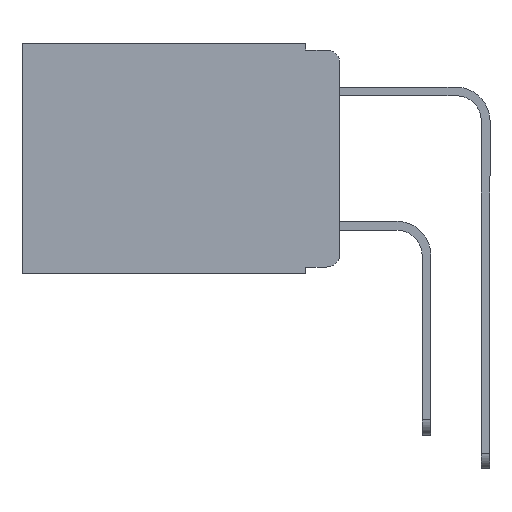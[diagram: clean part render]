
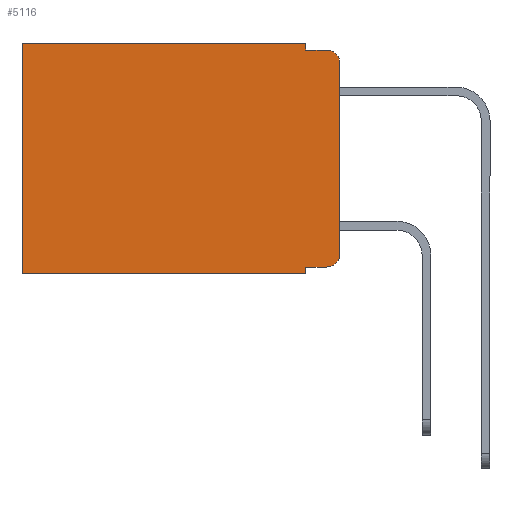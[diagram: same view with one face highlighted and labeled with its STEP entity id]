
A CAD part, left-side view. The second image highlights one B-rep face of the part: STEP entity #5116.
In plain terms, the highlighted planar face has unit normal (-1, 0, 0).
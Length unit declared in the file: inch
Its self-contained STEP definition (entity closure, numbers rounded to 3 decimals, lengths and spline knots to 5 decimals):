
#113 = EDGE_LOOP ( 'NONE', ( #5442, #7482, #9654, #10211, #340, #6336, #5883, #1117, #10622, #8975 ) ) ;
#290 = CARTESIAN_POINT ( 'NONE',  ( 0.298, 0.02, -0.333 ) ) ;
#305 = DIRECTION ( 'NONE',  ( 0., 0., -1. ) ) ;
#340 = ORIENTED_EDGE ( 'NONE', *, *, #9689, .T. ) ;
#457 = VERTEX_POINT ( 'NONE', #6332 ) ;
#502 = VERTEX_POINT ( 'NONE', #6420 ) ;
#534 = DIRECTION ( 'NONE',  ( 0., 1., 0. ) ) ;
#562 = CARTESIAN_POINT ( 'NONE',  ( 0.298, 0., -0.03 ) ) ;
#563 = CARTESIAN_POINT ( 'NONE',  ( 0.298, 0.051, -0.333 ) ) ;
#743 = VERTEX_POINT ( 'NONE', #6463 ) ;
#768 = LINE ( 'NONE', #3056, #7172 ) ;
#877 = EDGE_CURVE ( 'NONE', #502, #5134, #11701, .T. ) ;
#897 = VECTOR ( 'NONE', #6826, 39.37008 ) ;
#1117 = ORIENTED_EDGE ( 'NONE', *, *, #3532, .F. ) ;
#1133 = CARTESIAN_POINT ( 'NONE',  ( 0.298, 0., 0. ) ) ;
#1364 = LINE ( 'NONE', #2669, #6128 ) ;
#1477 = EDGE_CURVE ( 'NONE', #457, #4027, #4713, .T. ) ;
#1612 = CARTESIAN_POINT ( 'NONE',  ( 0.298, 0.051, -0.343 ) ) ;
#1953 = VECTOR ( 'NONE', #305, 39.37008 ) ;
#2151 = VECTOR ( 'NONE', #3379, 39.37008 ) ;
#2497 = VECTOR ( 'NONE', #5616, 39.37008 ) ;
#2669 = CARTESIAN_POINT ( 'NONE',  ( 0.298, 0., 0. ) ) ;
#2787 = VERTEX_POINT ( 'NONE', #6822 ) ;
#2798 = CARTESIAN_POINT ( 'NONE',  ( 0.298, 0.051, -0.01 ) ) ;
#3056 = CARTESIAN_POINT ( 'NONE',  ( 0.298, 0., -0.343 ) ) ;
#3106 = EDGE_CURVE ( 'NONE', #4027, #3108, #3943, .T. ) ;
#3108 = VERTEX_POINT ( 'NONE', #7665 ) ;
#3379 = DIRECTION ( 'NONE',  ( 0., 0., -1. ) ) ;
#3387 = VERTEX_POINT ( 'NONE', #562 ) ;
#3487 = LINE ( 'NONE', #1133, #897 ) ;
#3532 = EDGE_CURVE ( 'NONE', #502, #3729, #7193, .T. ) ;
#3574 = CARTESIAN_POINT ( 'NONE',  ( 0.298, 0.051, 0. ) ) ;
#3729 = VERTEX_POINT ( 'NONE', #1612 ) ;
#3780 = EDGE_CURVE ( 'NONE', #3387, #3108, #3946, .T. ) ;
#3943 = LINE ( 'NONE', #8588, #4243 ) ;
#3946 = CIRCLE ( 'NONE', #4612, 0.02 ) ;
#4027 = VERTEX_POINT ( 'NONE', #2798 ) ;
#4214 = LINE ( 'NONE', #4513, #1953 ) ;
#4243 = VECTOR ( 'NONE', #4510, 39.37008 ) ;
#4350 = PLANE ( 'NONE',  #9108 ) ;
#4391 = EDGE_CURVE ( 'NONE', #3729, #743, #768, .T. ) ;
#4510 = DIRECTION ( 'NONE',  ( 0., -1., 0. ) ) ;
#4513 = CARTESIAN_POINT ( 'NONE',  ( 0.298, 0.473, 0. ) ) ;
#4612 = AXIS2_PLACEMENT_3D ( 'NONE', #8884, #8831, #8600 ) ;
#4713 = LINE ( 'NONE', #4967, #2497 ) ;
#4967 = CARTESIAN_POINT ( 'NONE',  ( 0.298, 0.051, 0. ) ) ;
#5116 = ADVANCED_FACE ( 'NONE', ( #9204 ), #4350, .F. ) ;
#5117 = EDGE_CURVE ( 'NONE', #2787, #743, #4214, .T. ) ;
#5124 = CARTESIAN_POINT ( 'NONE',  ( 0.298, 0.02, -0.313 ) ) ;
#5134 = VERTEX_POINT ( 'NONE', #290 ) ;
#5442 = ORIENTED_EDGE ( 'NONE', *, *, #9468, .F. ) ;
#5616 = DIRECTION ( 'NONE',  ( 0., 0., -1. ) ) ;
#5821 = EDGE_CURVE ( 'NONE', #5134, #8566, #8761, .T. ) ;
#5883 = ORIENTED_EDGE ( 'NONE', *, *, #4391, .F. ) ;
#5899 = DIRECTION ( 'NONE',  ( 0., 0., -1. ) ) ;
#6081 = DIRECTION ( 'NONE',  ( 0., 0., -1. ) ) ;
#6128 = VECTOR ( 'NONE', #9274, 39.37008 ) ;
#6332 = CARTESIAN_POINT ( 'NONE',  ( 0.298, 0.051, 0. ) ) ;
#6336 = ORIENTED_EDGE ( 'NONE', *, *, #5117, .T. ) ;
#6420 = CARTESIAN_POINT ( 'NONE',  ( 0.298, 0.051, -0.333 ) ) ;
#6463 = CARTESIAN_POINT ( 'NONE',  ( 0.298, 0.473, -0.343 ) ) ;
#6745 = AXIS2_PLACEMENT_3D ( 'NONE', #5124, #11482, #6081 ) ;
#6822 = CARTESIAN_POINT ( 'NONE',  ( 0.298, 0.473, 0. ) ) ;
#6826 = DIRECTION ( 'NONE',  ( 0., 1., 0. ) ) ;
#6975 = CARTESIAN_POINT ( 'NONE',  ( 0.298, 0., -0.313 ) ) ;
#7172 = VECTOR ( 'NONE', #534, 39.37008 ) ;
#7193 = LINE ( 'NONE', #3574, #2151 ) ;
#7482 = ORIENTED_EDGE ( 'NONE', *, *, #3780, .T. ) ;
#7665 = CARTESIAN_POINT ( 'NONE',  ( 0.298, 0.02, -0.01 ) ) ;
#7922 = CARTESIAN_POINT ( 'NONE',  ( 0.298, 0., 0. ) ) ;
#8109 = DIRECTION ( 'NONE',  ( 0., -1., 0. ) ) ;
#8139 = DIRECTION ( 'NONE',  ( 1., 0., 0. ) ) ;
#8566 = VERTEX_POINT ( 'NONE', #6975 ) ;
#8588 = CARTESIAN_POINT ( 'NONE',  ( 0.298, 0.051, -0.01 ) ) ;
#8600 = DIRECTION ( 'NONE',  ( 0., 0., -1. ) ) ;
#8761 = CIRCLE ( 'NONE', #6745, 0.02 ) ;
#8831 = DIRECTION ( 'NONE',  ( -1., 0., 0. ) ) ;
#8884 = CARTESIAN_POINT ( 'NONE',  ( 0.298, 0.02, -0.03 ) ) ;
#8975 = ORIENTED_EDGE ( 'NONE', *, *, #5821, .T. ) ;
#9108 = AXIS2_PLACEMENT_3D ( 'NONE', #7922, #8139, #5899 ) ;
#9204 = FACE_OUTER_BOUND ( 'NONE', #113, .T. ) ;
#9274 = DIRECTION ( 'NONE',  ( 0., 0., -1. ) ) ;
#9406 = VECTOR ( 'NONE', #8109, 39.37008 ) ;
#9468 = EDGE_CURVE ( 'NONE', #3387, #8566, #1364, .T. ) ;
#9654 = ORIENTED_EDGE ( 'NONE', *, *, #3106, .F. ) ;
#9689 = EDGE_CURVE ( 'NONE', #457, #2787, #3487, .T. ) ;
#10211 = ORIENTED_EDGE ( 'NONE', *, *, #1477, .F. ) ;
#10622 = ORIENTED_EDGE ( 'NONE', *, *, #877, .T. ) ;
#11482 = DIRECTION ( 'NONE',  ( -1., 0., 0. ) ) ;
#11701 = LINE ( 'NONE', #563, #9406 ) ;
